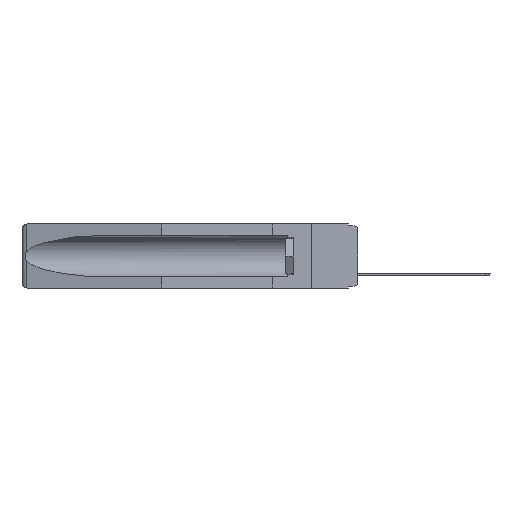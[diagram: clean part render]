
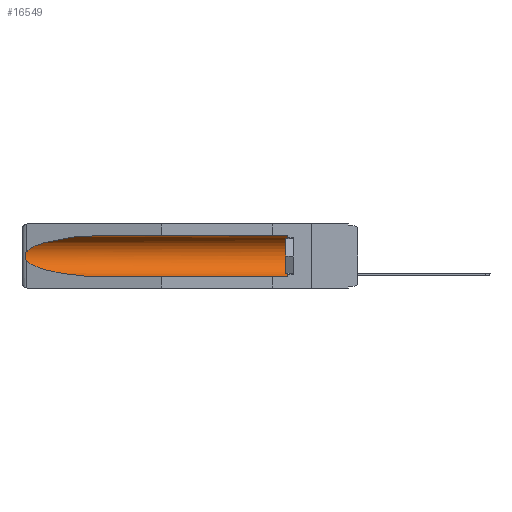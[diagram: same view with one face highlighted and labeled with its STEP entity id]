
A CAD part, left-side view. The second image highlights one B-rep face of the part: STEP entity #16549.
In plain terms, the highlighted cylindrical face has radius 2.857 mm (diameter 5.715 mm), a partial arc.
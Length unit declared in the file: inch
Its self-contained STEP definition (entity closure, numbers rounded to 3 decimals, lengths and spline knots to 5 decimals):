
#388 = CARTESIAN_POINT ( 'NONE',  ( 0.26537, 1.52718, -0.14972 ) ) ;
#485 = CARTESIAN_POINT ( 'NONE',  ( 0.155, 1.07973, -0.059 ) ) ;
#1049 = ORIENTED_EDGE ( 'NONE', *, *, #17013, .T. ) ;
#1574 = CARTESIAN_POINT ( 'NONE',  ( 0.26654, 1.53092, -0.15636 ) ) ;
#3371 = CARTESIAN_POINT ( 'NONE',  ( 0.26537, 1.52718, -0.19328 ) ) ;
#3769 = ORIENTED_EDGE ( 'NONE', *, *, #8637, .T. ) ;
#3851 =( BOUNDED_CURVE ( )  B_SPLINE_CURVE ( 3, ( #20475, #7517, #5724, #20572 ),
 .UNSPECIFIED., .F., .F. ) 
 B_SPLINE_CURVE_WITH_KNOTS ( ( 4, 4 ),
 ( 0.1948, 1.5708 ),
 .UNSPECIFIED. ) 
 CURVE ( )  GEOMETRIC_REPRESENTATION_ITEM ( )  RATIONAL_B_SPLINE_CURVE ( ( 1., 0.848, 0.848, 1. ) ) 
 REPRESENTATION_ITEM ( '' )  );
#4285 = ORIENTED_EDGE ( 'NONE', *, *, #13566, .F. ) ;
#4731 = CARTESIAN_POINT ( 'NONE',  ( 0.2675, 1.53308, -0.16763 ) ) ;
#4937 = CARTESIAN_POINT ( 'NONE',  ( 0.2673, 1.53269, -0.17917 ) ) ;
#5526 = CARTESIAN_POINT ( 'NONE',  ( 0.26537, 1.52718, -0.14972 ) ) ;
#5538 = CARTESIAN_POINT ( 'NONE',  ( 0.155, 1.07973, -0.284 ) ) ;
#5724 = CARTESIAN_POINT ( 'NONE',  ( 0.21114, 1.30732, -0.284 ) ) ;
#5985 = FACE_OUTER_BOUND ( 'NONE', #9713, .T. ) ;
#6151 = VERTEX_POINT ( 'NONE', #11763 ) ;
#7046 = VERTEX_POINT ( 'NONE', #20703 ) ;
#7179 = VERTEX_POINT ( 'NONE', #388 ) ;
#7495 = LINE ( 'NONE', #12242, #12619 ) ;
#7517 = CARTESIAN_POINT ( 'NONE',  ( 0.25451, 1.48313, -0.24835 ) ) ;
#8120 = CARTESIAN_POINT ( 'NONE',  ( 0.155, 0.126, -0.1715 ) ) ;
#8432 = VERTEX_POINT ( 'NONE', #17484 ) ;
#8637 = EDGE_CURVE ( 'NONE', #8432, #7179, #13879, .T. ) ;
#8927 = CARTESIAN_POINT ( 'NONE',  ( 0.155, -0.30754, -0.284 ) ) ;
#9079 = VECTOR ( 'NONE', #9244, 39.37008 ) ;
#9244 = DIRECTION ( 'NONE',  ( 0., 1., 0. ) ) ;
#9713 = EDGE_LOOP ( 'NONE', ( #3769, #16911, #1049, #4285, #12846, #14414 ) ) ;
#10627 = AXIS2_PLACEMENT_3D ( 'NONE', #13604, #18436, #10635 ) ;
#10635 = DIRECTION ( 'NONE',  ( 0., 0., 1. ) ) ;
#11008 = AXIS2_PLACEMENT_3D ( 'NONE', #8120, #15941, #19278 ) ;
#11051 = EDGE_CURVE ( 'NONE', #7046, #6151, #20078, .T. ) ;
#11763 = CARTESIAN_POINT ( 'NONE',  ( 0.155, 0.126, -0.059 ) ) ;
#12138 = B_SPLINE_CURVE_WITH_KNOTS ( 'NONE', 3,
 ( #15935, #14582, #1574, #19273, #4731, #14170, #4937, #12665, #17611, #3371 ),
 .UNSPECIFIED., .F., .F.,
 ( 4, 2, 2, 2, 4 ),
 ( 0., 0.00029, 0.00058, 0.00087, 0.00117 ),
 .UNSPECIFIED. ) ;
#12242 = CARTESIAN_POINT ( 'NONE',  ( 0.155, -0.30754, -0.059 ) ) ;
#12464 = DIRECTION ( 'NONE',  ( 0., 1., 0. ) ) ;
#12619 = VECTOR ( 'NONE', #12464, 39.37008 ) ;
#12665 = CARTESIAN_POINT ( 'NONE',  ( 0.26655, 1.53094, -0.18657 ) ) ;
#12846 = ORIENTED_EDGE ( 'NONE', *, *, #11051, .T. ) ;
#13566 = EDGE_CURVE ( 'NONE', #7046, #20322, #17076, .T. ) ;
#13604 = CARTESIAN_POINT ( 'NONE',  ( 0.155, -0.30754, -0.1715 ) ) ;
#13827 = CYLINDRICAL_SURFACE ( 'NONE', #10627, 0.1125 ) ;
#13879 =( BOUNDED_CURVE ( )  B_SPLINE_CURVE ( 3, ( #485, #19780, #18210, #5526 ),
 .UNSPECIFIED., .F., .F. ) 
 B_SPLINE_CURVE_WITH_KNOTS ( ( 4, 4 ),
 ( 4.71239, 6.08839 ),
 .UNSPECIFIED. ) 
 CURVE ( )  GEOMETRIC_REPRESENTATION_ITEM ( )  RATIONAL_B_SPLINE_CURVE ( ( 1., 0.848, 0.848, 1. ) ) 
 REPRESENTATION_ITEM ( '' )  );
#14170 = CARTESIAN_POINT ( 'NONE',  ( 0.2675, 1.53308, -0.17534 ) ) ;
#14414 = ORIENTED_EDGE ( 'NONE', *, *, #17363, .T. ) ;
#14582 = CARTESIAN_POINT ( 'NONE',  ( 0.26597, 1.52961, -0.15275 ) ) ;
#15935 = CARTESIAN_POINT ( 'NONE',  ( 0.26537, 1.52718, -0.14972 ) ) ;
#15941 = DIRECTION ( 'NONE',  ( 0., -1., 0. ) ) ;
#16279 = EDGE_CURVE ( 'NONE', #7179, #17401, #12138, .T. ) ;
#16549 = ADVANCED_FACE ( 'NONE', ( #5985 ), #13827, .F. ) ;
#16911 = ORIENTED_EDGE ( 'NONE', *, *, #16279, .T. ) ;
#17013 = EDGE_CURVE ( 'NONE', #17401, #20322, #3851, .T. ) ;
#17076 = LINE ( 'NONE', #8927, #9079 ) ;
#17363 = EDGE_CURVE ( 'NONE', #6151, #8432, #7495, .T. ) ;
#17401 = VERTEX_POINT ( 'NONE', #20449 ) ;
#17484 = CARTESIAN_POINT ( 'NONE',  ( 0.155, 1.07973, -0.059 ) ) ;
#17611 = CARTESIAN_POINT ( 'NONE',  ( 0.26597, 1.5296, -0.19026 ) ) ;
#18210 = CARTESIAN_POINT ( 'NONE',  ( 0.25451, 1.48313, -0.09465 ) ) ;
#18436 = DIRECTION ( 'NONE',  ( 0., 1., 0. ) ) ;
#19273 = CARTESIAN_POINT ( 'NONE',  ( 0.2673, 1.5327, -0.16383 ) ) ;
#19278 = DIRECTION ( 'NONE',  ( 0., 0., 1. ) ) ;
#19780 = CARTESIAN_POINT ( 'NONE',  ( 0.21114, 1.30732, -0.059 ) ) ;
#20078 = CIRCLE ( 'NONE', #11008, 0.1125 ) ;
#20322 = VERTEX_POINT ( 'NONE', #5538 ) ;
#20449 = CARTESIAN_POINT ( 'NONE',  ( 0.26537, 1.52718, -0.19328 ) ) ;
#20475 = CARTESIAN_POINT ( 'NONE',  ( 0.26537, 1.52718, -0.19328 ) ) ;
#20572 = CARTESIAN_POINT ( 'NONE',  ( 0.155, 1.07973, -0.284 ) ) ;
#20703 = CARTESIAN_POINT ( 'NONE',  ( 0.155, 0.126, -0.284 ) ) ;
